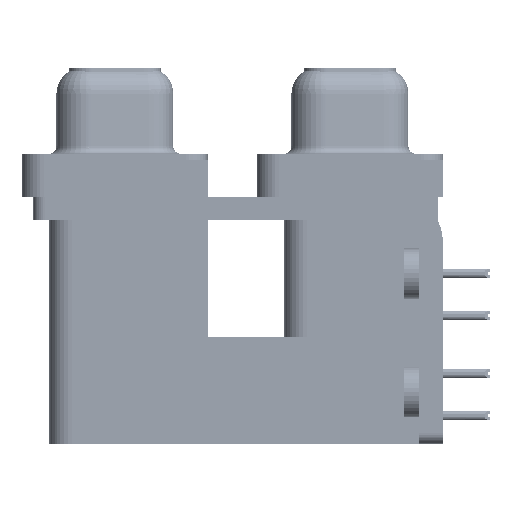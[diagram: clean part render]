
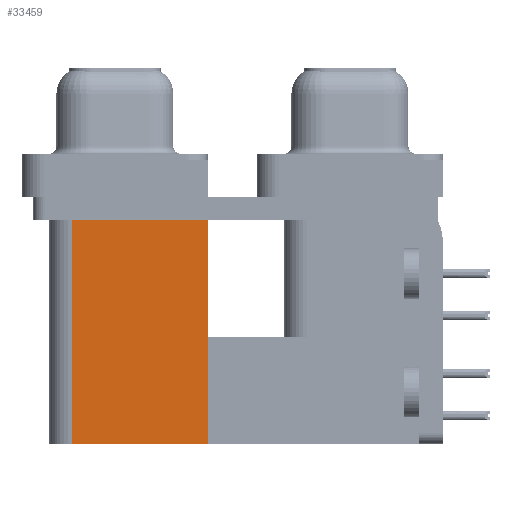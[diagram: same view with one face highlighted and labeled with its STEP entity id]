
A CAD part, left-side view. The second image highlights one B-rep face of the part: STEP entity #33459.
In plain terms, the highlighted planar face has unit normal (-1, 0, 0).
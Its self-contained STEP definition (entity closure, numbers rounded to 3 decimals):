
#1561 = VERTEX_POINT ( 'NONE', #44465 ) ;
#2415 = DIRECTION ( 'NONE',  ( 0., 0., 1. ) ) ;
#3511 = VECTOR ( 'NONE', #2415, 1000. ) ;
#5848 = VECTOR ( 'NONE', #13035, 1000. ) ;
#6758 = CARTESIAN_POINT ( 'NONE',  ( 3.79, 9.6, -19.2 ) ) ;
#8850 = LINE ( 'NONE', #74149, #22056 ) ;
#9235 = VERTEX_POINT ( 'NONE', #13212 ) ;
#13035 = DIRECTION ( 'NONE',  ( 0., 1., 0. ) ) ;
#13212 = CARTESIAN_POINT ( 'NONE',  ( 3.79, 18.8, -19.2 ) ) ;
#14068 = LINE ( 'NONE', #37007, #26161 ) ;
#19081 = ORIENTED_EDGE ( 'NONE', *, *, #56782, .T. ) ;
#19668 = ORIENTED_EDGE ( 'NONE', *, *, #47596, .F. ) ;
#20886 = DIRECTION ( 'NONE',  ( 0., 1., 0. ) ) ;
#22056 = VECTOR ( 'NONE', #20886, 1000. ) ;
#22320 = VERTEX_POINT ( 'NONE', #28551 ) ;
#25082 = VERTEX_POINT ( 'NONE', #69190 ) ;
#26161 = VECTOR ( 'NONE', #55652, 1000. ) ;
#28551 = CARTESIAN_POINT ( 'NONE',  ( 3.79, 18.8, -2.5 ) ) ;
#30482 = DIRECTION ( 'NONE',  ( 1., 0., 0. ) ) ;
#33459 = ADVANCED_FACE ( 'NONE', ( #53821 ), #60010, .F. ) ;
#37007 = CARTESIAN_POINT ( 'NONE',  ( 3.79, 9.6, -19.2 ) ) ;
#43665 = LINE ( 'NONE', #56826, #3511 ) ;
#44465 = CARTESIAN_POINT ( 'NONE',  ( 3.79, 9.6, -19.2 ) ) ;
#47596 = EDGE_CURVE ( 'NONE', #1561, #9235, #71373, .T. ) ;
#48787 = EDGE_CURVE ( 'NONE', #25082, #22320, #8850, .T. ) ;
#49128 = EDGE_CURVE ( 'NONE', #9235, #22320, #43665, .T. ) ;
#53821 = FACE_OUTER_BOUND ( 'NONE', #69796, .T. ) ;
#54184 = DIRECTION ( 'NONE',  ( 0., 0., -1. ) ) ;
#55652 = DIRECTION ( 'NONE',  ( 0., 0., 1. ) ) ;
#56782 = EDGE_CURVE ( 'NONE', #1561, #25082, #14068, .T. ) ;
#56826 = CARTESIAN_POINT ( 'NONE',  ( 3.79, 18.8, -19.2 ) ) ;
#58366 = ORIENTED_EDGE ( 'NONE', *, *, #48787, .T. ) ;
#60010 = PLANE ( 'NONE',  #61139 ) ;
#60648 = ORIENTED_EDGE ( 'NONE', *, *, #49128, .F. ) ;
#61139 = AXIS2_PLACEMENT_3D ( 'NONE', #6758, #30482, #54184 ) ;
#66293 = CARTESIAN_POINT ( 'NONE',  ( 3.79, 9.6, -19.2 ) ) ;
#69190 = CARTESIAN_POINT ( 'NONE',  ( 3.79, 9.6, -2.5 ) ) ;
#69796 = EDGE_LOOP ( 'NONE', ( #58366, #60648, #19668, #19081 ) ) ;
#71373 = LINE ( 'NONE', #66293, #5848 ) ;
#74149 = CARTESIAN_POINT ( 'NONE',  ( 3.79, 9.6, -2.5 ) ) ;
